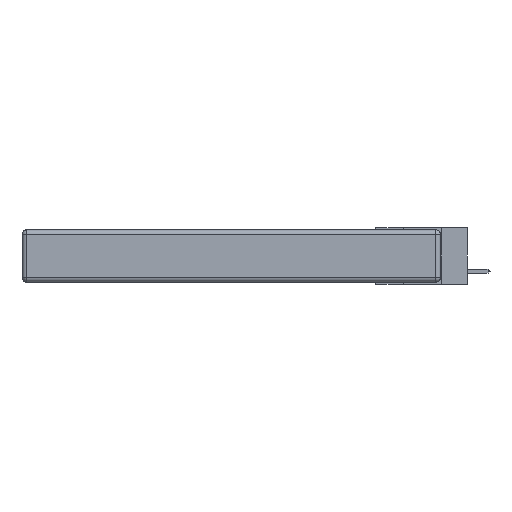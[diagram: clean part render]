
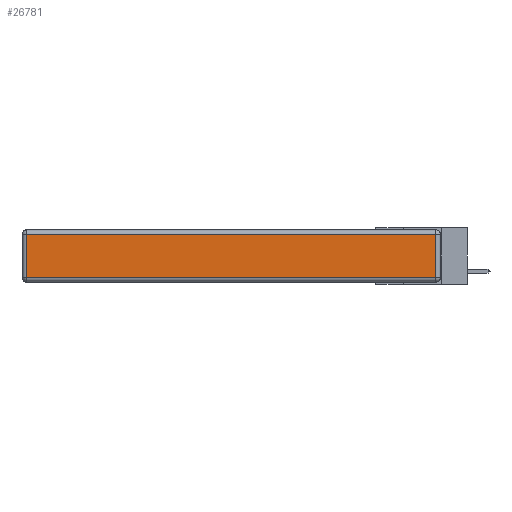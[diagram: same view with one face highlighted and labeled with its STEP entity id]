
A CAD part, left-side view. The second image highlights one B-rep face of the part: STEP entity #26781.
In plain terms, the highlighted planar face has unit normal (-1, 0, 0).
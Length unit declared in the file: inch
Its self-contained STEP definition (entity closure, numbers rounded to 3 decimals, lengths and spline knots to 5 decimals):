
#2582 = LINE ( 'NONE', #19287, #26319 ) ;
#2784 = FACE_OUTER_BOUND ( 'NONE', #6569, .T. ) ;
#2973 = DIRECTION ( 'NONE',  ( 0., 0., 1. ) ) ;
#3156 = CARTESIAN_POINT ( 'NONE',  ( 0., 0.03, -0.03 ) ) ;
#3603 = DIRECTION ( 'NONE',  ( 0., -1., 0. ) ) ;
#4057 = ORIENTED_EDGE ( 'NONE', *, *, #16087, .T. ) ;
#4341 = CARTESIAN_POINT ( 'NONE',  ( 0., 2.72, -0.03 ) ) ;
#4974 = DIRECTION ( 'NONE',  ( -1., 0., 0. ) ) ;
#6012 = EDGE_CURVE ( 'NONE', #8141, #7746, #2582, .T. ) ;
#6218 = CARTESIAN_POINT ( 'NONE',  ( 0., 2.72, -0.313 ) ) ;
#6569 = EDGE_LOOP ( 'NONE', ( #4057, #21351, #20079, #12185 ) ) ;
#7386 = PLANE ( 'NONE',  #7688 ) ;
#7688 = AXIS2_PLACEMENT_3D ( 'NONE', #9807, #4974, #2973 ) ;
#7746 = VERTEX_POINT ( 'NONE', #4341 ) ;
#7922 = CARTESIAN_POINT ( 'NONE',  ( 0., 0., -0.313 ) ) ;
#8141 = VERTEX_POINT ( 'NONE', #3156 ) ;
#9807 = CARTESIAN_POINT ( 'NONE',  ( 0., 0., -0.343 ) ) ;
#9817 = CARTESIAN_POINT ( 'NONE',  ( 0., 2.72, -0.343 ) ) ;
#12185 = ORIENTED_EDGE ( 'NONE', *, *, #12336, .T. ) ;
#12336 = EDGE_CURVE ( 'NONE', #7746, #24898, #17522, .T. ) ;
#13144 = LINE ( 'NONE', #7922, #21077 ) ;
#15370 = CARTESIAN_POINT ( 'NONE',  ( 0., 0.03, -0.343 ) ) ;
#15675 = EDGE_CURVE ( 'NONE', #25264, #8141, #19808, .T. ) ;
#16087 = EDGE_CURVE ( 'NONE', #24898, #25264, #13144, .T. ) ;
#17522 = LINE ( 'NONE', #9817, #23626 ) ;
#18723 = VECTOR ( 'NONE', #19817, 39.37008 ) ;
#19287 = CARTESIAN_POINT ( 'NONE',  ( 0., 2.75, -0.03 ) ) ;
#19808 = LINE ( 'NONE', #15370, #18723 ) ;
#19817 = DIRECTION ( 'NONE',  ( 0., 0., 1. ) ) ;
#20079 = ORIENTED_EDGE ( 'NONE', *, *, #6012, .T. ) ;
#21076 = DIRECTION ( 'NONE',  ( 0., 0., -1. ) ) ;
#21077 = VECTOR ( 'NONE', #3603, 39.37008 ) ;
#21351 = ORIENTED_EDGE ( 'NONE', *, *, #15675, .T. ) ;
#23626 = VECTOR ( 'NONE', #21076, 39.37008 ) ;
#23802 = DIRECTION ( 'NONE',  ( 0., 1., 0. ) ) ;
#24110 = CARTESIAN_POINT ( 'NONE',  ( 0., 0.03, -0.313 ) ) ;
#24898 = VERTEX_POINT ( 'NONE', #6218 ) ;
#25264 = VERTEX_POINT ( 'NONE', #24110 ) ;
#26319 = VECTOR ( 'NONE', #23802, 39.37008 ) ;
#26781 = ADVANCED_FACE ( 'NONE', ( #2784 ), #7386, .T. ) ;
